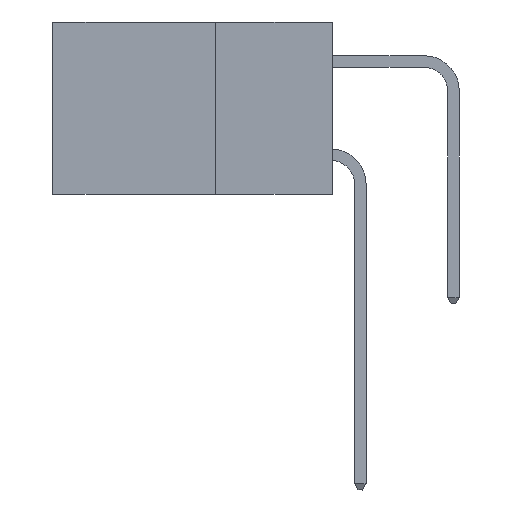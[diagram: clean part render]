
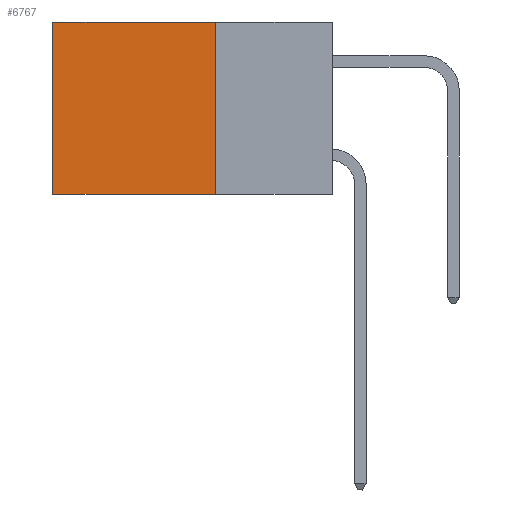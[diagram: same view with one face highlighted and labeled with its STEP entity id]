
A CAD part, left-side view. The second image highlights one B-rep face of the part: STEP entity #6767.
In plain terms, the highlighted planar face has unit normal (-1, 0, 0).
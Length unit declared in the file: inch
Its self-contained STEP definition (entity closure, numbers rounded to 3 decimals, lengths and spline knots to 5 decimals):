
#322 = VERTEX_POINT ( 'NONE', #11348 ) ;
#332 = DIRECTION ( 'NONE',  ( 0., 0., -1. ) ) ;
#779 = DIRECTION ( 'NONE',  ( 0., 0., -1. ) ) ;
#1021 = LINE ( 'NONE', #4609, #9489 ) ;
#1143 = ORIENTED_EDGE ( 'NONE', *, *, #7546, .F. ) ;
#1860 = CARTESIAN_POINT ( 'NONE',  ( 0.2615, 0.25, -0.37 ) ) ;
#3277 = EDGE_LOOP ( 'NONE', ( #11166, #1143, #5684, #7734 ) ) ;
#3424 = DIRECTION ( 'NONE',  ( 1., 0., 0. ) ) ;
#3429 = EDGE_CURVE ( 'NONE', #10952, #6507, #9006, .T. ) ;
#3729 = CARTESIAN_POINT ( 'NONE',  ( 0.2615, 0.6, 0. ) ) ;
#3945 = CARTESIAN_POINT ( 'NONE',  ( 0.2615, 0.6, -0.37 ) ) ;
#4357 = FACE_OUTER_BOUND ( 'NONE', #3277, .T. ) ;
#4467 = CARTESIAN_POINT ( 'NONE',  ( 0.2615, 0.25, 0. ) ) ;
#4609 = CARTESIAN_POINT ( 'NONE',  ( 0.2615, 0.25, -0.37 ) ) ;
#5217 = PLANE ( 'NONE',  #5416 ) ;
#5332 = DIRECTION ( 'NONE',  ( 0., 1., 0. ) ) ;
#5416 = AXIS2_PLACEMENT_3D ( 'NONE', #1860, #3424, #779 ) ;
#5564 = CARTESIAN_POINT ( 'NONE',  ( 0.2615, 0.25, -0.37 ) ) ;
#5684 = ORIENTED_EDGE ( 'NONE', *, *, #10393, .F. ) ;
#5963 = EDGE_CURVE ( 'NONE', #322, #10952, #8062, .T. ) ;
#6504 = DIRECTION ( 'NONE',  ( 0., 1., 0. ) ) ;
#6507 = VERTEX_POINT ( 'NONE', #11357 ) ;
#6767 = ADVANCED_FACE ( 'NONE', ( #4357 ), #5217, .F. ) ;
#6998 = DIRECTION ( 'NONE',  ( 0., 0., -1. ) ) ;
#7424 = VECTOR ( 'NONE', #6504, 39.37008 ) ;
#7546 = EDGE_CURVE ( 'NONE', #9066, #6507, #9077, .T. ) ;
#7734 = ORIENTED_EDGE ( 'NONE', *, *, #5963, .T. ) ;
#8062 = LINE ( 'NONE', #4467, #10180 ) ;
#9006 = LINE ( 'NONE', #3945, #10078 ) ;
#9066 = VERTEX_POINT ( 'NONE', #9276 ) ;
#9077 = LINE ( 'NONE', #5564, #7424 ) ;
#9276 = CARTESIAN_POINT ( 'NONE',  ( 0.2615, 0.25, -0.37 ) ) ;
#9489 = VECTOR ( 'NONE', #6998, 39.37008 ) ;
#10078 = VECTOR ( 'NONE', #332, 39.37008 ) ;
#10180 = VECTOR ( 'NONE', #5332, 39.37008 ) ;
#10393 = EDGE_CURVE ( 'NONE', #322, #9066, #1021, .T. ) ;
#10952 = VERTEX_POINT ( 'NONE', #3729 ) ;
#11166 = ORIENTED_EDGE ( 'NONE', *, *, #3429, .T. ) ;
#11348 = CARTESIAN_POINT ( 'NONE',  ( 0.2615, 0.25, 0. ) ) ;
#11357 = CARTESIAN_POINT ( 'NONE',  ( 0.2615, 0.6, -0.37 ) ) ;
